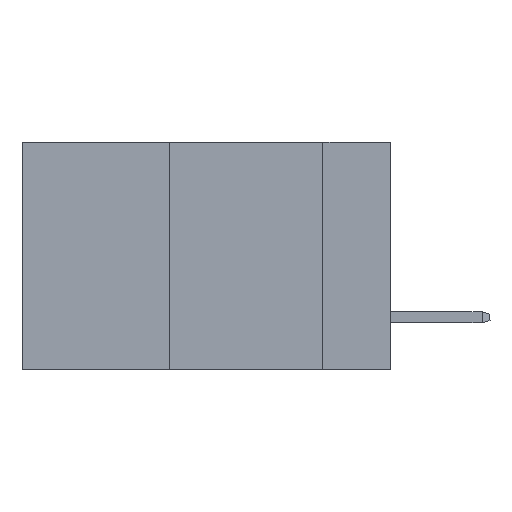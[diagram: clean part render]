
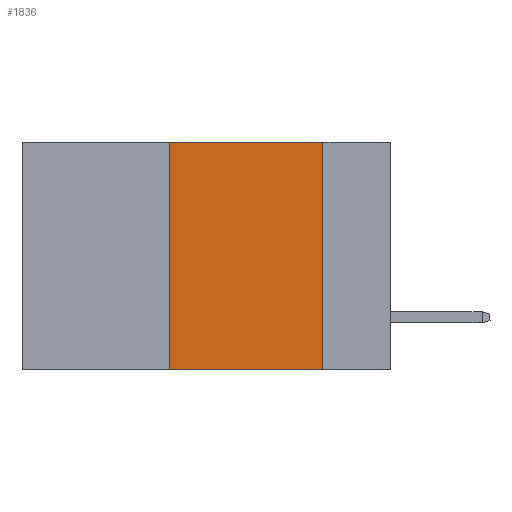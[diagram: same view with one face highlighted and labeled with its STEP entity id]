
A CAD part, left-side view. The second image highlights one B-rep face of the part: STEP entity #1836.
In plain terms, the highlighted planar face has unit normal (-1, 0, 0).
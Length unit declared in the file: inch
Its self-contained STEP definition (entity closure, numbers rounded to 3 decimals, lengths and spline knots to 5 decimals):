
#17 = DIRECTION ( 'NONE',  ( 0., -1., 0. ) ) ;
#1017 = VERTEX_POINT ( 'NONE', #16845 ) ;
#1390 = LINE ( 'NONE', #4810, #10049 ) ;
#1836 = ADVANCED_FACE ( 'NONE', ( #8918 ), #4637, .F. ) ;
#2450 = VERTEX_POINT ( 'NONE', #14951 ) ;
#3017 = VECTOR ( 'NONE', #17, 39.37008 ) ;
#3189 = VERTEX_POINT ( 'NONE', #21786 ) ;
#3218 = VERTEX_POINT ( 'NONE', #10519 ) ;
#4552 = CARTESIAN_POINT ( 'NONE',  ( 0., 0.6, 0. ) ) ;
#4637 = PLANE ( 'NONE',  #17829 ) ;
#4645 = DIRECTION ( 'NONE',  ( 0., 0., 1. ) ) ;
#4810 = CARTESIAN_POINT ( 'NONE',  ( 0., 0.6, -0.37 ) ) ;
#6212 = CARTESIAN_POINT ( 'NONE',  ( 0., 0.11, 0. ) ) ;
#6748 = ORIENTED_EDGE ( 'NONE', *, *, #24764, .F. ) ;
#6943 = LINE ( 'NONE', #6212, #16027 ) ;
#8918 = FACE_OUTER_BOUND ( 'NONE', #23054, .T. ) ;
#10049 = VECTOR ( 'NONE', #14552, 39.37008 ) ;
#10519 = CARTESIAN_POINT ( 'NONE',  ( 0., 0.36, -0.37 ) ) ;
#11265 = ORIENTED_EDGE ( 'NONE', *, *, #18081, .F. ) ;
#11860 = LINE ( 'NONE', #16313, #16389 ) ;
#12134 = EDGE_CURVE ( 'NONE', #3218, #3189, #11860, .T. ) ;
#12188 = EDGE_CURVE ( 'NONE', #3218, #1017, #1390, .T. ) ;
#13435 = LINE ( 'NONE', #17641, #3017 ) ;
#14552 = DIRECTION ( 'NONE',  ( 0., -1., 0. ) ) ;
#14951 = CARTESIAN_POINT ( 'NONE',  ( 0., 0.11, 0. ) ) ;
#16027 = VECTOR ( 'NONE', #21555, 39.37008 ) ;
#16313 = CARTESIAN_POINT ( 'NONE',  ( 0., 0.36, 0. ) ) ;
#16389 = VECTOR ( 'NONE', #4645, 39.37008 ) ;
#16845 = CARTESIAN_POINT ( 'NONE',  ( 0., 0.11, -0.37 ) ) ;
#17010 = ORIENTED_EDGE ( 'NONE', *, *, #12134, .F. ) ;
#17580 = ORIENTED_EDGE ( 'NONE', *, *, #12188, .T. ) ;
#17641 = CARTESIAN_POINT ( 'NONE',  ( 0., 0.6, 0. ) ) ;
#17829 = AXIS2_PLACEMENT_3D ( 'NONE', #4552, #23821, #22610 ) ;
#18081 = EDGE_CURVE ( 'NONE', #2450, #1017, #6943, .T. ) ;
#21555 = DIRECTION ( 'NONE',  ( 0., 0., -1. ) ) ;
#21786 = CARTESIAN_POINT ( 'NONE',  ( 0., 0.36, 0. ) ) ;
#22610 = DIRECTION ( 'NONE',  ( 0., 0., -1. ) ) ;
#23054 = EDGE_LOOP ( 'NONE', ( #11265, #6748, #17010, #17580 ) ) ;
#23821 = DIRECTION ( 'NONE',  ( 1., 0., 0. ) ) ;
#24764 = EDGE_CURVE ( 'NONE', #3189, #2450, #13435, .T. ) ;
